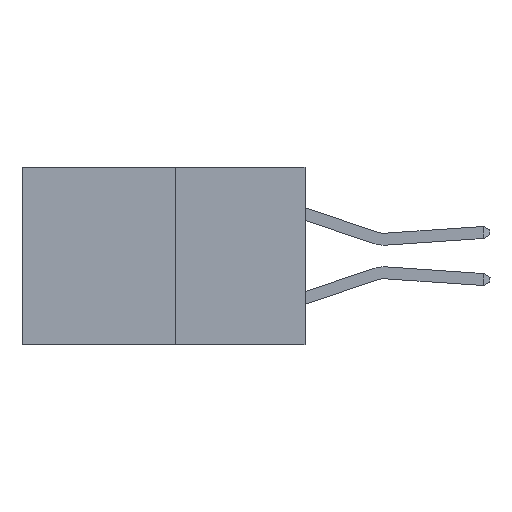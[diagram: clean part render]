
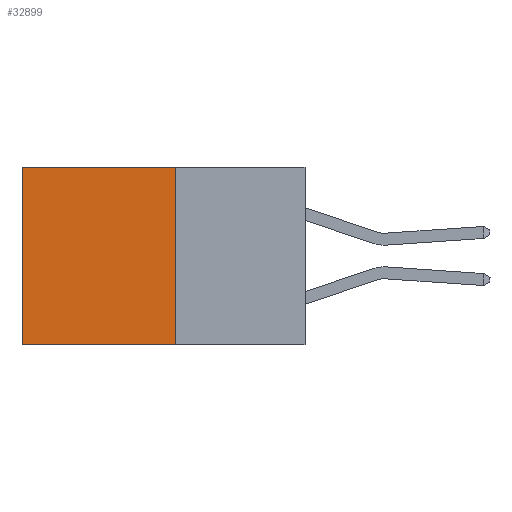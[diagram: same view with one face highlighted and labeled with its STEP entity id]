
A CAD part, left-side view. The second image highlights one B-rep face of the part: STEP entity #32899.
In plain terms, the highlighted planar face has unit normal (-1, 0, 0).
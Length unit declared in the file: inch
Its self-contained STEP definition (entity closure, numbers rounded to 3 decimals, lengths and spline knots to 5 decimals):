
#330 = VECTOR ( 'NONE', #25304, 39.37008 ) ;
#3620 = CARTESIAN_POINT ( 'NONE',  ( 0.277, 0.59, 0. ) ) ;
#4483 = DIRECTION ( 'NONE',  ( 0., 0., -1. ) ) ;
#5023 = CARTESIAN_POINT ( 'NONE',  ( 0.277, 0.27, -0.37 ) ) ;
#5076 = ORIENTED_EDGE ( 'NONE', *, *, #32225, .F. ) ;
#5661 = CARTESIAN_POINT ( 'NONE',  ( 0.277, 0.59, -0.37 ) ) ;
#8758 = VERTEX_POINT ( 'NONE', #5023 ) ;
#9099 = EDGE_CURVE ( 'NONE', #19646, #15150, #14294, .T. ) ;
#9196 = EDGE_CURVE ( 'NONE', #8758, #24335, #11863, .T. ) ;
#10168 = FACE_OUTER_BOUND ( 'NONE', #20594, .T. ) ;
#11006 = VECTOR ( 'NONE', #23030, 39.37008 ) ;
#11863 = LINE ( 'NONE', #23103, #11006 ) ;
#11955 = LINE ( 'NONE', #30421, #31906 ) ;
#14294 = LINE ( 'NONE', #25767, #330 ) ;
#15150 = VERTEX_POINT ( 'NONE', #3620 ) ;
#16745 = VECTOR ( 'NONE', #25565, 39.37008 ) ;
#17433 = DIRECTION ( 'NONE',  ( 0., 0., -1. ) ) ;
#17541 = CARTESIAN_POINT ( 'NONE',  ( 0.277, 0.27, -0.37 ) ) ;
#18874 = ORIENTED_EDGE ( 'NONE', *, *, #9099, .T. ) ;
#19646 = VERTEX_POINT ( 'NONE', #31381 ) ;
#20132 = DIRECTION ( 'NONE',  ( 1., 0., 0. ) ) ;
#20594 = EDGE_LOOP ( 'NONE', ( #28009, #30689, #5076, #18874 ) ) ;
#22947 = CARTESIAN_POINT ( 'NONE',  ( 0.277, 0.27, -0.37 ) ) ;
#23030 = DIRECTION ( 'NONE',  ( 0., 1., 0. ) ) ;
#23089 = AXIS2_PLACEMENT_3D ( 'NONE', #17541, #20132, #4483 ) ;
#23103 = CARTESIAN_POINT ( 'NONE',  ( 0.277, 0.27, -0.37 ) ) ;
#24335 = VERTEX_POINT ( 'NONE', #5661 ) ;
#25304 = DIRECTION ( 'NONE',  ( 0., 1., 0. ) ) ;
#25565 = DIRECTION ( 'NONE',  ( 0., 0., -1. ) ) ;
#25766 = EDGE_CURVE ( 'NONE', #15150, #24335, #11955, .T. ) ;
#25767 = CARTESIAN_POINT ( 'NONE',  ( 0.277, 0.27, 0. ) ) ;
#28009 = ORIENTED_EDGE ( 'NONE', *, *, #25766, .T. ) ;
#30421 = CARTESIAN_POINT ( 'NONE',  ( 0.277, 0.59, -0.37 ) ) ;
#30689 = ORIENTED_EDGE ( 'NONE', *, *, #9196, .F. ) ;
#31381 = CARTESIAN_POINT ( 'NONE',  ( 0.277, 0.27, 0. ) ) ;
#31441 = LINE ( 'NONE', #22947, #16745 ) ;
#31906 = VECTOR ( 'NONE', #17433, 39.37008 ) ;
#32225 = EDGE_CURVE ( 'NONE', #19646, #8758, #31441, .T. ) ;
#32899 = ADVANCED_FACE ( 'NONE', ( #10168 ), #33137, .F. ) ;
#33137 = PLANE ( 'NONE',  #23089 ) ;
